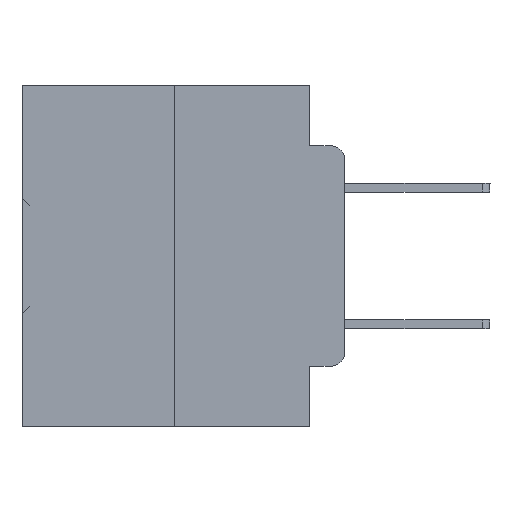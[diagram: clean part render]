
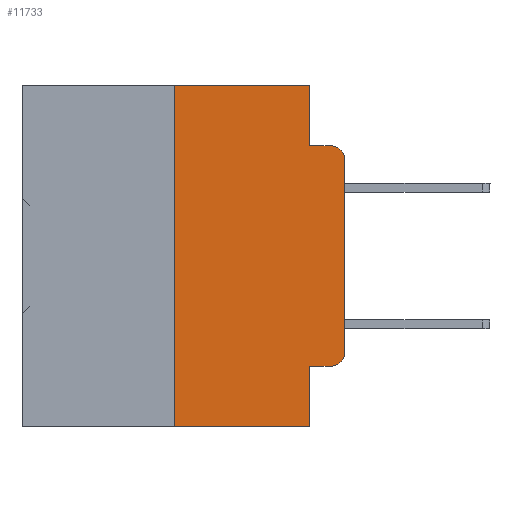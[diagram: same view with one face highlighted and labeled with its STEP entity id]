
A CAD part, left-side view. The second image highlights one B-rep face of the part: STEP entity #11733.
In plain terms, the highlighted planar face has unit normal (-1, 0, 0).
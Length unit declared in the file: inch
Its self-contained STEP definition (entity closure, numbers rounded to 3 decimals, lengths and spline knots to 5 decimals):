
#934 = VECTOR ( 'NONE', #28815, 39.37008 ) ;
#1411 = DIRECTION ( 'NONE',  ( 0., 0., 1. ) ) ;
#1490 = CARTESIAN_POINT ( 'NONE',  ( 0., 0.051, -0.0885 ) ) ;
#1613 = DIRECTION ( 'NONE',  ( 0., -1., 0. ) ) ;
#2858 = VECTOR ( 'NONE', #1613, 39.37008 ) ;
#2901 = VECTOR ( 'NONE', #13205, 39.37008 ) ;
#2905 = DIRECTION ( 'NONE',  ( -1., 0., 0. ) ) ;
#3031 = DIRECTION ( 'NONE',  ( 0., 0., -1. ) ) ;
#3420 = DIRECTION ( 'NONE',  ( 0., -1., 0. ) ) ;
#3682 = ORIENTED_EDGE ( 'NONE', *, *, #18022, .F. ) ;
#3749 = EDGE_LOOP ( 'NONE', ( #24655, #17648, #33983, #28852, #3682, #14114, #12441, #10912, #10362, #37951 ) ) ;
#3830 = LINE ( 'NONE', #35911, #17813 ) ;
#5367 = VERTEX_POINT ( 'NONE', #17115 ) ;
#5476 = CARTESIAN_POINT ( 'NONE',  ( 0., 0.02, -0.3915 ) ) ;
#5486 = EDGE_CURVE ( 'NONE', #24998, #36268, #14562, .T. ) ;
#6892 = AXIS2_PLACEMENT_3D ( 'NONE', #22746, #22497, #13779 ) ;
#7530 = LINE ( 'NONE', #22305, #30813 ) ;
#7546 = DIRECTION ( 'NONE',  ( 0., -1., 0. ) ) ;
#7864 = AXIS2_PLACEMENT_3D ( 'NONE', #14854, #2905, #3031 ) ;
#8458 = LINE ( 'NONE', #33883, #2901 ) ;
#9846 = CARTESIAN_POINT ( 'NONE',  ( 0., 0.051, 0. ) ) ;
#10362 = ORIENTED_EDGE ( 'NONE', *, *, #17247, .T. ) ;
#10601 = EDGE_CURVE ( 'NONE', #12956, #12032, #8458, .T. ) ;
#10912 = ORIENTED_EDGE ( 'NONE', *, *, #22901, .F. ) ;
#11399 = CARTESIAN_POINT ( 'NONE',  ( 0., 0.051, -0.4115 ) ) ;
#11733 = ADVANCED_FACE ( 'NONE', ( #15809 ), #13396, .F. ) ;
#11924 = EDGE_CURVE ( 'NONE', #5367, #18508, #36272, .T. ) ;
#12032 = VERTEX_POINT ( 'NONE', #36886 ) ;
#12291 = VERTEX_POINT ( 'NONE', #11399 ) ;
#12441 = ORIENTED_EDGE ( 'NONE', *, *, #28522, .T. ) ;
#12956 = VERTEX_POINT ( 'NONE', #9846 ) ;
#13196 = CARTESIAN_POINT ( 'NONE',  ( 0., 0., -0.3915 ) ) ;
#13205 = DIRECTION ( 'NONE',  ( 0., 0., -1. ) ) ;
#13396 = PLANE ( 'NONE',  #6892 ) ;
#13477 = VERTEX_POINT ( 'NONE', #13196 ) ;
#13779 = DIRECTION ( 'NONE',  ( 0., 0., -1. ) ) ;
#13872 = CARTESIAN_POINT ( 'NONE',  ( 0., 0.02, -0.0885 ) ) ;
#14114 = ORIENTED_EDGE ( 'NONE', *, *, #11924, .F. ) ;
#14327 = LINE ( 'NONE', #1490, #35748 ) ;
#14562 = CIRCLE ( 'NONE', #7864, 0.02 ) ;
#14854 = CARTESIAN_POINT ( 'NONE',  ( 0., 0.02, -0.1085 ) ) ;
#15809 = FACE_OUTER_BOUND ( 'NONE', #3749, .T. ) ;
#15979 = CARTESIAN_POINT ( 'NONE',  ( 0., 0.02, -0.4115 ) ) ;
#17115 = CARTESIAN_POINT ( 'NONE',  ( 0., 0.25, -0.5 ) ) ;
#17247 = EDGE_CURVE ( 'NONE', #12291, #31109, #3830, .T. ) ;
#17648 = ORIENTED_EDGE ( 'NONE', *, *, #5486, .T. ) ;
#17813 = VECTOR ( 'NONE', #3420, 39.37008 ) ;
#18022 = EDGE_CURVE ( 'NONE', #18508, #12956, #29846, .T. ) ;
#18066 = DIRECTION ( 'NONE',  ( 0., 0., -1. ) ) ;
#18508 = VERTEX_POINT ( 'NONE', #21932 ) ;
#18585 = AXIS2_PLACEMENT_3D ( 'NONE', #5476, #35239, #29425 ) ;
#19422 = VERTEX_POINT ( 'NONE', #28419 ) ;
#19675 = VECTOR ( 'NONE', #7546, 39.37008 ) ;
#20006 = EDGE_CURVE ( 'NONE', #12032, #36268, #14327, .T. ) ;
#20138 = EDGE_CURVE ( 'NONE', #31109, #13477, #36202, .T. ) ;
#21932 = CARTESIAN_POINT ( 'NONE',  ( 0., 0.25, 0. ) ) ;
#22251 = CARTESIAN_POINT ( 'NONE',  ( 0., 0.473, 0. ) ) ;
#22305 = CARTESIAN_POINT ( 'NONE',  ( 0., 0., 0. ) ) ;
#22497 = DIRECTION ( 'NONE',  ( 1., 0., 0. ) ) ;
#22746 = CARTESIAN_POINT ( 'NONE',  ( 0., 0.473, 0. ) ) ;
#22901 = EDGE_CURVE ( 'NONE', #12291, #19422, #34190, .T. ) ;
#24212 = EDGE_CURVE ( 'NONE', #13477, #24998, #7530, .T. ) ;
#24655 = ORIENTED_EDGE ( 'NONE', *, *, #24212, .T. ) ;
#24998 = VERTEX_POINT ( 'NONE', #35253 ) ;
#25810 = VECTOR ( 'NONE', #18066, 39.37008 ) ;
#28262 = DIRECTION ( 'NONE',  ( 0., -1., 0. ) ) ;
#28419 = CARTESIAN_POINT ( 'NONE',  ( 0., 0.051, -0.5 ) ) ;
#28522 = EDGE_CURVE ( 'NONE', #5367, #19422, #29521, .T. ) ;
#28815 = DIRECTION ( 'NONE',  ( 0., 0., 1. ) ) ;
#28852 = ORIENTED_EDGE ( 'NONE', *, *, #10601, .F. ) ;
#29425 = DIRECTION ( 'NONE',  ( 0., 0., -1. ) ) ;
#29521 = LINE ( 'NONE', #37239, #19675 ) ;
#29846 = LINE ( 'NONE', #22251, #2858 ) ;
#30813 = VECTOR ( 'NONE', #1411, 39.37008 ) ;
#31109 = VERTEX_POINT ( 'NONE', #15979 ) ;
#33883 = CARTESIAN_POINT ( 'NONE',  ( 0., 0.051, 0. ) ) ;
#33983 = ORIENTED_EDGE ( 'NONE', *, *, #20006, .F. ) ;
#34190 = LINE ( 'NONE', #35856, #25810 ) ;
#35239 = DIRECTION ( 'NONE',  ( -1., 0., 0. ) ) ;
#35253 = CARTESIAN_POINT ( 'NONE',  ( 0., 0., -0.1085 ) ) ;
#35748 = VECTOR ( 'NONE', #28262, 39.37008 ) ;
#35856 = CARTESIAN_POINT ( 'NONE',  ( 0., 0.051, 0. ) ) ;
#35911 = CARTESIAN_POINT ( 'NONE',  ( 0., 0.051, -0.4115 ) ) ;
#36202 = CIRCLE ( 'NONE', #18585, 0.02 ) ;
#36268 = VERTEX_POINT ( 'NONE', #13872 ) ;
#36272 = LINE ( 'NONE', #36775, #934 ) ;
#36775 = CARTESIAN_POINT ( 'NONE',  ( 0., 0.25, 0. ) ) ;
#36886 = CARTESIAN_POINT ( 'NONE',  ( 0., 0.051, -0.0885 ) ) ;
#37239 = CARTESIAN_POINT ( 'NONE',  ( 0., 0.473, -0.5 ) ) ;
#37951 = ORIENTED_EDGE ( 'NONE', *, *, #20138, .T. ) ;
